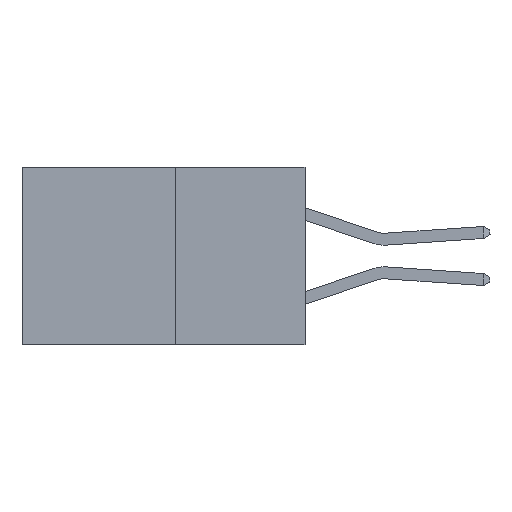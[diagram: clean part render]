
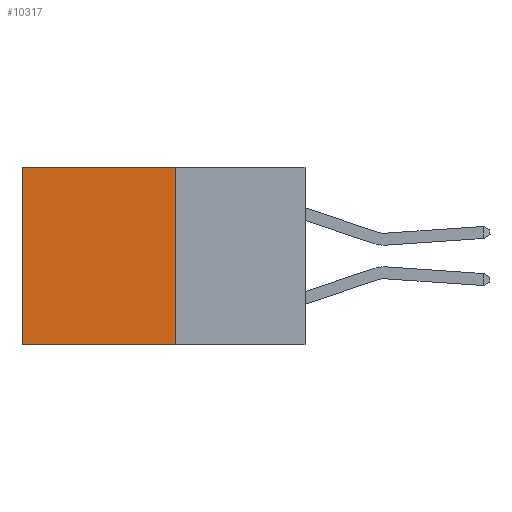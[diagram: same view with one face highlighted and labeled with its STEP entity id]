
A CAD part, left-side view. The second image highlights one B-rep face of the part: STEP entity #10317.
In plain terms, the highlighted planar face has unit normal (-1, 0, 0).
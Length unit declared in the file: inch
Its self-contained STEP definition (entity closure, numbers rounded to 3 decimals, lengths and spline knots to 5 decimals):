
#134 = LINE ( 'NONE', #10967, #15630 ) ;
#274 = CARTESIAN_POINT ( 'NONE',  ( 0.277, 0.27, 0. ) ) ;
#788 = VERTEX_POINT ( 'NONE', #10002 ) ;
#2805 = ORIENTED_EDGE ( 'NONE', *, *, #5930, .F. ) ;
#3622 = LINE ( 'NONE', #6892, #11402 ) ;
#4426 = DIRECTION ( 'NONE',  ( 1., 0., 0. ) ) ;
#5656 = EDGE_CURVE ( 'NONE', #15550, #788, #16844, .T. ) ;
#5930 = EDGE_CURVE ( 'NONE', #8950, #788, #134, .T. ) ;
#6538 = ORIENTED_EDGE ( 'NONE', *, *, #7461, .F. ) ;
#6892 = CARTESIAN_POINT ( 'NONE',  ( 0.277, 0.27, 0. ) ) ;
#7461 = EDGE_CURVE ( 'NONE', #8791, #8950, #13160, .T. ) ;
#8268 = ORIENTED_EDGE ( 'NONE', *, *, #11438, .T. ) ;
#8791 = VERTEX_POINT ( 'NONE', #274 ) ;
#8950 = VERTEX_POINT ( 'NONE', #10637 ) ;
#9681 = DIRECTION ( 'NONE',  ( 0., 0., -1. ) ) ;
#9991 = VECTOR ( 'NONE', #9681, 39.37008 ) ;
#10002 = CARTESIAN_POINT ( 'NONE',  ( 0.277, 0.59, -0.37 ) ) ;
#10317 = ADVANCED_FACE ( 'NONE', ( #12187 ), #13715, .F. ) ;
#10468 = CARTESIAN_POINT ( 'NONE',  ( 0.277, 0.27, -0.37 ) ) ;
#10637 = CARTESIAN_POINT ( 'NONE',  ( 0.277, 0.27, -0.37 ) ) ;
#10967 = CARTESIAN_POINT ( 'NONE',  ( 0.277, 0.27, -0.37 ) ) ;
#10987 = DIRECTION ( 'NONE',  ( 0., 1., 0. ) ) ;
#11402 = VECTOR ( 'NONE', #11578, 39.37008 ) ;
#11438 = EDGE_CURVE ( 'NONE', #8791, #15550, #3622, .T. ) ;
#11578 = DIRECTION ( 'NONE',  ( 0., 1., 0. ) ) ;
#12157 = CARTESIAN_POINT ( 'NONE',  ( 0.277, 0.27, -0.37 ) ) ;
#12187 = FACE_OUTER_BOUND ( 'NONE', #17002, .T. ) ;
#12743 = VECTOR ( 'NONE', #13894, 39.37008 ) ;
#13160 = LINE ( 'NONE', #10468, #9991 ) ;
#13715 = PLANE ( 'NONE',  #14315 ) ;
#13894 = DIRECTION ( 'NONE',  ( 0., 0., -1. ) ) ;
#14120 = CARTESIAN_POINT ( 'NONE',  ( 0.277, 0.59, -0.37 ) ) ;
#14315 = AXIS2_PLACEMENT_3D ( 'NONE', #12157, #4426, #15265 ) ;
#15012 = CARTESIAN_POINT ( 'NONE',  ( 0.277, 0.59, 0. ) ) ;
#15265 = DIRECTION ( 'NONE',  ( 0., 0., -1. ) ) ;
#15550 = VERTEX_POINT ( 'NONE', #15012 ) ;
#15630 = VECTOR ( 'NONE', #10987, 39.37008 ) ;
#16844 = LINE ( 'NONE', #14120, #12743 ) ;
#17002 = EDGE_LOOP ( 'NONE', ( #19173, #2805, #6538, #8268 ) ) ;
#19173 = ORIENTED_EDGE ( 'NONE', *, *, #5656, .T. ) ;
